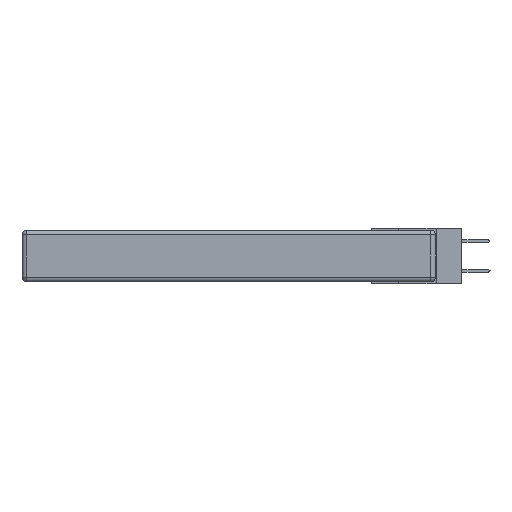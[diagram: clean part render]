
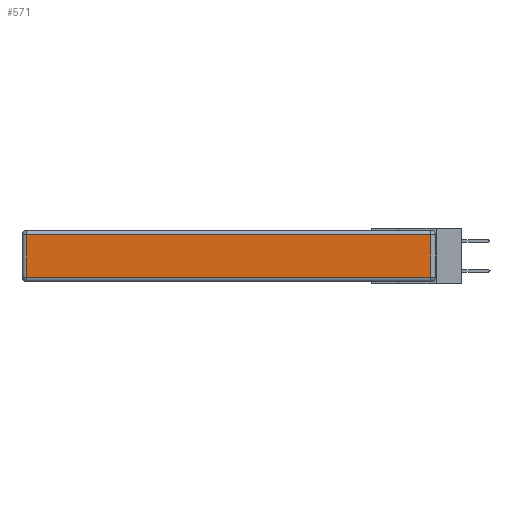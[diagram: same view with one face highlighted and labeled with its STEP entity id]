
A CAD part, left-side view. The second image highlights one B-rep face of the part: STEP entity #571.
In plain terms, the highlighted planar face has unit normal (-1, 0, 0).
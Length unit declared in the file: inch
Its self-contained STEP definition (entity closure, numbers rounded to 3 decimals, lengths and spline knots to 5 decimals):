
#402 = CARTESIAN_POINT ( 'NONE',  ( 0., 0.03, -0.313 ) ) ;
#542 = CARTESIAN_POINT ( 'NONE',  ( 0., 0.03, -0.03 ) ) ;
#571 = ADVANCED_FACE ( 'NONE', ( #3289 ), #13329, .T. ) ;
#776 = AXIS2_PLACEMENT_3D ( 'NONE', #14636, #1986, #1843 ) ;
#1219 = EDGE_CURVE ( 'NONE', #7360, #2642, #8316, .T. ) ;
#1843 = DIRECTION ( 'NONE',  ( 0., 0., 1. ) ) ;
#1986 = DIRECTION ( 'NONE',  ( -1., 0., 0. ) ) ;
#2208 = VECTOR ( 'NONE', #12721, 39.37008 ) ;
#2642 = VERTEX_POINT ( 'NONE', #402 ) ;
#2995 = DIRECTION ( 'NONE',  ( 0., 0., -1. ) ) ;
#3055 = VERTEX_POINT ( 'NONE', #542 ) ;
#3289 = FACE_OUTER_BOUND ( 'NONE', #9562, .T. ) ;
#4420 = EDGE_CURVE ( 'NONE', #2642, #3055, #6679, .T. ) ;
#4727 = CARTESIAN_POINT ( 'NONE',  ( 0., 0.03, -0.343 ) ) ;
#5216 = VECTOR ( 'NONE', #12815, 39.37008 ) ;
#5809 = LINE ( 'NONE', #10006, #11573 ) ;
#6558 = VECTOR ( 'NONE', #6643, 39.37008 ) ;
#6643 = DIRECTION ( 'NONE',  ( 0., 1., 0. ) ) ;
#6679 = LINE ( 'NONE', #4727, #5216 ) ;
#6984 = CARTESIAN_POINT ( 'NONE',  ( 0., 0., -0.313 ) ) ;
#7360 = VERTEX_POINT ( 'NONE', #12131 ) ;
#7759 = ORIENTED_EDGE ( 'NONE', *, *, #10826, .T. ) ;
#8316 = LINE ( 'NONE', #6984, #2208 ) ;
#8346 = LINE ( 'NONE', #13525, #6558 ) ;
#9562 = EDGE_LOOP ( 'NONE', ( #12324, #13633, #14913, #7759 ) ) ;
#10006 = CARTESIAN_POINT ( 'NONE',  ( 0., 2.72, -0.343 ) ) ;
#10826 = EDGE_CURVE ( 'NONE', #11395, #7360, #5809, .T. ) ;
#11395 = VERTEX_POINT ( 'NONE', #13745 ) ;
#11573 = VECTOR ( 'NONE', #2995, 39.37008 ) ;
#12131 = CARTESIAN_POINT ( 'NONE',  ( 0., 2.72, -0.313 ) ) ;
#12324 = ORIENTED_EDGE ( 'NONE', *, *, #1219, .T. ) ;
#12662 = EDGE_CURVE ( 'NONE', #3055, #11395, #8346, .T. ) ;
#12721 = DIRECTION ( 'NONE',  ( 0., -1., 0. ) ) ;
#12815 = DIRECTION ( 'NONE',  ( 0., 0., 1. ) ) ;
#13329 = PLANE ( 'NONE',  #776 ) ;
#13525 = CARTESIAN_POINT ( 'NONE',  ( 0., 2.75, -0.03 ) ) ;
#13633 = ORIENTED_EDGE ( 'NONE', *, *, #4420, .T. ) ;
#13745 = CARTESIAN_POINT ( 'NONE',  ( 0., 2.72, -0.03 ) ) ;
#14636 = CARTESIAN_POINT ( 'NONE',  ( 0., 0., -0.343 ) ) ;
#14913 = ORIENTED_EDGE ( 'NONE', *, *, #12662, .T. ) ;
